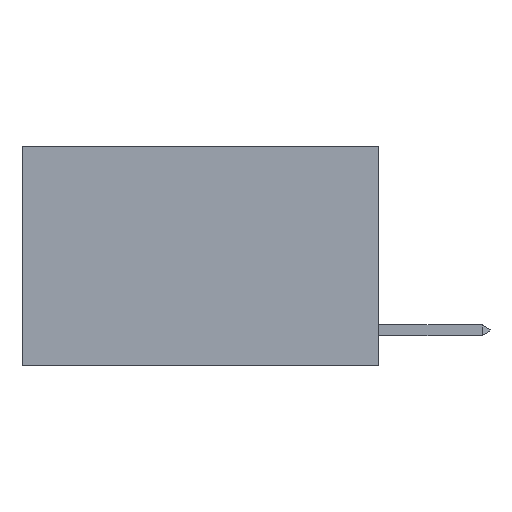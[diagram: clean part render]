
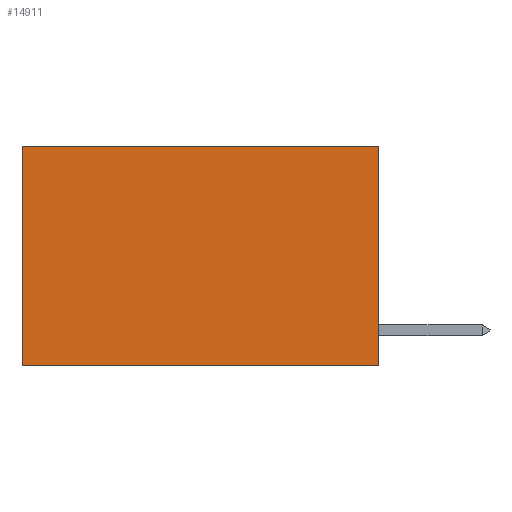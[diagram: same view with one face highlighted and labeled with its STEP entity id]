
A CAD part, left-side view. The second image highlights one B-rep face of the part: STEP entity #14911.
In plain terms, the highlighted planar face has unit normal (-1, 0, 0).
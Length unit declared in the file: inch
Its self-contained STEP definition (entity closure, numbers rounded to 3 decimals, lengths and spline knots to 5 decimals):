
#195 = VECTOR ( 'NONE', #12945, 39.37008 ) ;
#396 = CARTESIAN_POINT ( 'NONE',  ( 0.2625, 0.6, 0. ) ) ;
#1358 = AXIS2_PLACEMENT_3D ( 'NONE', #4261, #10555, #3019 ) ;
#1769 = DIRECTION ( 'NONE',  ( 0., 0., -1. ) ) ;
#1835 = VERTEX_POINT ( 'NONE', #15737 ) ;
#2321 = LINE ( 'NONE', #11848, #11957 ) ;
#2454 = EDGE_CURVE ( 'NONE', #2468, #1835, #12580, .T. ) ;
#2468 = VERTEX_POINT ( 'NONE', #9353 ) ;
#2705 = ORIENTED_EDGE ( 'NONE', *, *, #13329, .F. ) ;
#3019 = DIRECTION ( 'NONE',  ( 0., 0., -1. ) ) ;
#3148 = EDGE_LOOP ( 'NONE', ( #11881, #4123, #2705, #5513 ) ) ;
#3478 = DIRECTION ( 'NONE',  ( 0., 1., 0. ) ) ;
#3624 = LINE ( 'NONE', #396, #195 ) ;
#4123 = ORIENTED_EDGE ( 'NONE', *, *, #15488, .F. ) ;
#4261 = CARTESIAN_POINT ( 'NONE',  ( 0.2625, 0., 0. ) ) ;
#5113 = CARTESIAN_POINT ( 'NONE',  ( 0.2625, 0., 0. ) ) ;
#5513 = ORIENTED_EDGE ( 'NONE', *, *, #2454, .T. ) ;
#6816 = PLANE ( 'NONE',  #1358 ) ;
#7302 = CARTESIAN_POINT ( 'NONE',  ( 0.2625, 0.6, -0.37 ) ) ;
#8319 = VERTEX_POINT ( 'NONE', #7302 ) ;
#9353 = CARTESIAN_POINT ( 'NONE',  ( 0.2625, 0., 0. ) ) ;
#9691 = VECTOR ( 'NONE', #3478, 39.37008 ) ;
#10555 = DIRECTION ( 'NONE',  ( 1., 0., 0. ) ) ;
#11848 = CARTESIAN_POINT ( 'NONE',  ( 0.2625, 0., 0. ) ) ;
#11881 = ORIENTED_EDGE ( 'NONE', *, *, #16024, .T. ) ;
#11884 = VECTOR ( 'NONE', #11902, 39.37008 ) ;
#11902 = DIRECTION ( 'NONE',  ( 0., 1., 0. ) ) ;
#11957 = VECTOR ( 'NONE', #1769, 39.37008 ) ;
#12262 = LINE ( 'NONE', #13063, #11884 ) ;
#12288 = VERTEX_POINT ( 'NONE', #13294 ) ;
#12580 = LINE ( 'NONE', #5113, #9691 ) ;
#12945 = DIRECTION ( 'NONE',  ( 0., 0., -1. ) ) ;
#13063 = CARTESIAN_POINT ( 'NONE',  ( 0.2625, 0., -0.37 ) ) ;
#13294 = CARTESIAN_POINT ( 'NONE',  ( 0.2625, 0., -0.37 ) ) ;
#13329 = EDGE_CURVE ( 'NONE', #2468, #12288, #2321, .T. ) ;
#13802 = FACE_OUTER_BOUND ( 'NONE', #3148, .T. ) ;
#14911 = ADVANCED_FACE ( 'NONE', ( #13802 ), #6816, .F. ) ;
#15488 = EDGE_CURVE ( 'NONE', #12288, #8319, #12262, .T. ) ;
#15737 = CARTESIAN_POINT ( 'NONE',  ( 0.2625, 0.6, 0. ) ) ;
#16024 = EDGE_CURVE ( 'NONE', #1835, #8319, #3624, .T. ) ;
